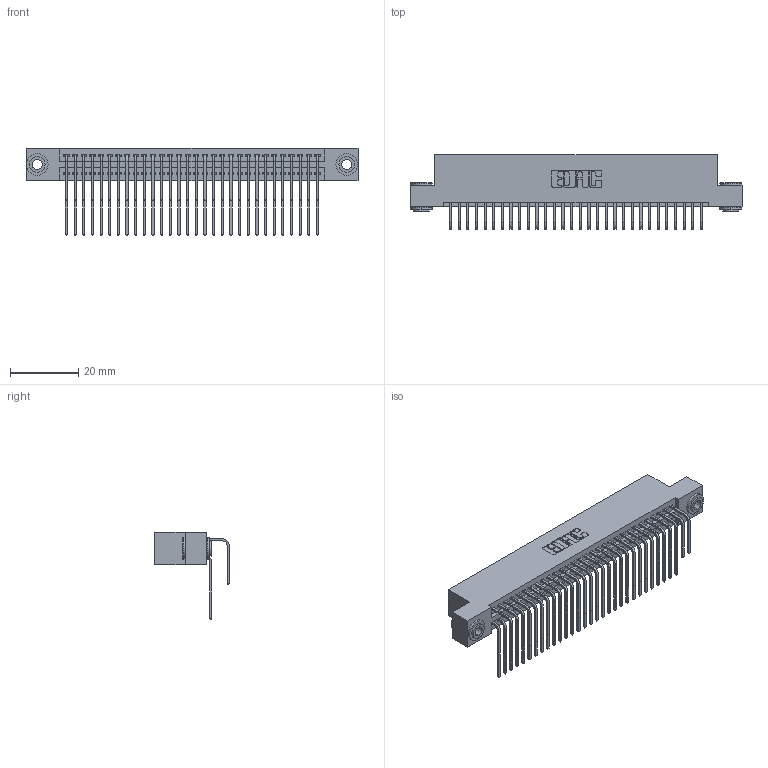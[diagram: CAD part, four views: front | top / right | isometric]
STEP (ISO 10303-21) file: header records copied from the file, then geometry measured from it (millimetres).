
FILE_DESCRIPTION (( 'STEP AP203' ), '1' );
FILE_NAME ('395-060-558-203.STEP', '2019-10-23T14:51:45', ( '' ), ( '' ), 'SwSTEP 2.0', 'SolidWorks 2016', '' );
FILE_SCHEMA (( 'CONFIG_CONTROL_DESIGN' ));
Length unit declared in the file: inch
Products named in the file (5): 345 Part_Flush Mounting Lugs - 0.156 Dia-TH; 345-292-001_558 559 Tail - 1; 345-292-001_558 Tail - 2; 345-250-002_345-250-002-102; 395-060-558-203
Assembly tree (63 placements, depth 2):
  395-060-558-203
    345 Part_Flush Mounting Lugs - 0.156 Dia-TH
    345-292-001_558 559 Tail - 1  x30
    345-292-001_558 Tail - 2  x30
    345-250-002_345-250-002-102  x2
Bounding box: 97.41 x 21.83 x 25.53 mm (x, y, z)
Volume: 9716.5 mm3; surface area: 15962.7 mm2
Topology: 63 solids, 63 shells, 3284 faces, 9717 edges, 6394 vertices
Faces by surface type: plane 2190, cylinder 1086, cone 8
Entity records: 27456 total; most frequent: CARTESIAN_POINT 4634, ORIENTED_EDGE 4510, DIRECTION 4105, EDGE_CURVE 2255, VECTOR 1939, LINE 1939, VERTEX_POINT 1498, AXIS2_PLACEMENT_3D 1083
